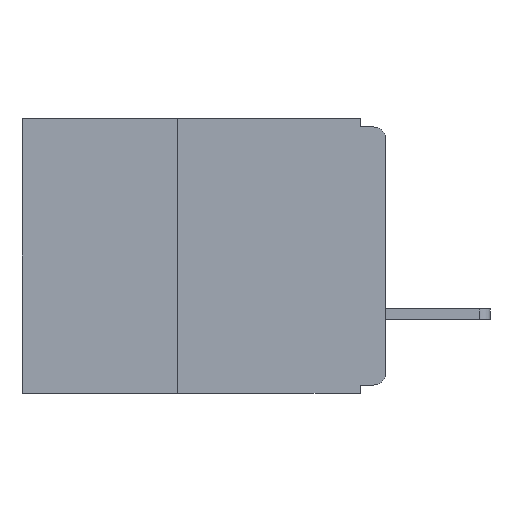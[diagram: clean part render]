
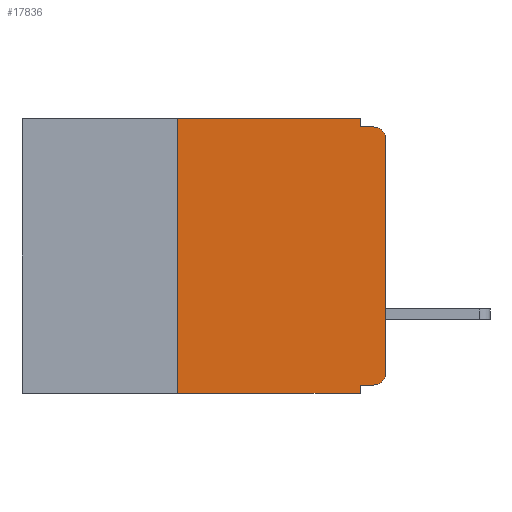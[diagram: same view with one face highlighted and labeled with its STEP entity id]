
A CAD part, left-side view. The second image highlights one B-rep face of the part: STEP entity #17836.
In plain terms, the highlighted planar face has unit normal (-1, 0, 0).
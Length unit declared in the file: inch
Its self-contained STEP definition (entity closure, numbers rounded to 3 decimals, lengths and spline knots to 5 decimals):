
#217 = ORIENTED_EDGE ( 'NONE', *, *, #17724, .F. ) ;
#242 = ORIENTED_EDGE ( 'NONE', *, *, #21918, .T. ) ;
#341 = ORIENTED_EDGE ( 'NONE', *, *, #3918, .T. ) ;
#465 = ORIENTED_EDGE ( 'NONE', *, *, #1792, .T. ) ;
#536 = VECTOR ( 'NONE', #16294, 39.37008 ) ;
#741 = ORIENTED_EDGE ( 'NONE', *, *, #10838, .F. ) ;
#824 = LINE ( 'NONE', #5973, #21567 ) ;
#985 = ORIENTED_EDGE ( 'NONE', *, *, #1573, .F. ) ;
#1011 = VERTEX_POINT ( 'NONE', #6963 ) ;
#1187 = ORIENTED_EDGE ( 'NONE', *, *, #6076, .T. ) ;
#1283 = ORIENTED_EDGE ( 'NONE', *, *, #16368, .F. ) ;
#1501 = DIRECTION ( 'NONE',  ( 0., 0., -1. ) ) ;
#1509 = DIRECTION ( 'NONE',  ( -1., 0., 0. ) ) ;
#1535 = CARTESIAN_POINT ( 'NONE',  ( 0., 0.015, -0.305 ) ) ;
#1573 = EDGE_CURVE ( 'NONE', #5684, #25303, #824, .T. ) ;
#1792 = EDGE_CURVE ( 'NONE', #17069, #1011, #11176, .T. ) ;
#2097 = DIRECTION ( 'NONE',  ( 0., 0., -1. ) ) ;
#2385 = LINE ( 'NONE', #5655, #23067 ) ;
#2975 = VECTOR ( 'NONE', #23339, 39.37008 ) ;
#3246 = VECTOR ( 'NONE', #16067, 39.37008 ) ;
#3507 = CARTESIAN_POINT ( 'NONE',  ( 0., 0., -0.025 ) ) ;
#3577 = CARTESIAN_POINT ( 'NONE',  ( 0., 0., -0.305 ) ) ;
#3665 = EDGE_CURVE ( 'NONE', #7034, #17385, #2385, .T. ) ;
#3918 = EDGE_CURVE ( 'NONE', #24389, #17069, #22154, .T. ) ;
#4003 = PLANE ( 'NONE',  #12230 ) ;
#4044 = CARTESIAN_POINT ( 'NONE',  ( 0., 0.031, -0.33 ) ) ;
#4451 = DIRECTION ( 'NONE',  ( 1., 0., 0. ) ) ;
#4988 = VERTEX_POINT ( 'NONE', #16734 ) ;
#5291 = CARTESIAN_POINT ( 'NONE',  ( 0., 0., -0.01 ) ) ;
#5655 = CARTESIAN_POINT ( 'NONE',  ( 0., 0.031, 0. ) ) ;
#5684 = VERTEX_POINT ( 'NONE', #5942 ) ;
#5814 = DIRECTION ( 'NONE',  ( 0., -1., 0. ) ) ;
#5861 = LINE ( 'NONE', #10238, #536 ) ;
#5942 = CARTESIAN_POINT ( 'NONE',  ( 0., 0.015, -0.32 ) ) ;
#5973 = CARTESIAN_POINT ( 'NONE',  ( 0., 0., -0.32 ) ) ;
#6076 = EDGE_CURVE ( 'NONE', #5684, #24389, #23247, .T. ) ;
#6673 = VECTOR ( 'NONE', #7690, 39.37008 ) ;
#6963 = CARTESIAN_POINT ( 'NONE',  ( 0., 0.015, -0.01 ) ) ;
#7034 = VERTEX_POINT ( 'NONE', #23872 ) ;
#7690 = DIRECTION ( 'NONE',  ( 0., 0., 1. ) ) ;
#8330 = EDGE_LOOP ( 'NONE', ( #341, #465, #1283, #15384, #20646, #217, #242, #741, #985, #1187 ) ) ;
#8595 = LINE ( 'NONE', #4044, #3246 ) ;
#8597 = CARTESIAN_POINT ( 'NONE',  ( 0., 0.031, -0.01 ) ) ;
#8864 = FACE_OUTER_BOUND ( 'NONE', #8330, .T. ) ;
#9011 = EDGE_CURVE ( 'NONE', #11824, #7034, #5861, .T. ) ;
#10238 = CARTESIAN_POINT ( 'NONE',  ( 0., 0.437, 0. ) ) ;
#10838 = EDGE_CURVE ( 'NONE', #25303, #16185, #8595, .T. ) ;
#10985 = DIRECTION ( 'NONE',  ( 0., 1., 0. ) ) ;
#11176 = CIRCLE ( 'NONE', #24838, 0.015 ) ;
#11362 = LINE ( 'NONE', #21753, #6673 ) ;
#11824 = VERTEX_POINT ( 'NONE', #21210 ) ;
#12105 = VECTOR ( 'NONE', #16089, 39.37008 ) ;
#12230 = AXIS2_PLACEMENT_3D ( 'NONE', #16493, #4451, #18567 ) ;
#13435 = AXIS2_PLACEMENT_3D ( 'NONE', #1535, #1509, #1501 ) ;
#15027 = CARTESIAN_POINT ( 'NONE',  ( 0., 0.031, -0.32 ) ) ;
#15384 = ORIENTED_EDGE ( 'NONE', *, *, #3665, .F. ) ;
#16067 = DIRECTION ( 'NONE',  ( 0., 0., -1. ) ) ;
#16089 = DIRECTION ( 'NONE',  ( 0., 0., 1. ) ) ;
#16185 = VERTEX_POINT ( 'NONE', #20790 ) ;
#16294 = DIRECTION ( 'NONE',  ( 0., -1., 0. ) ) ;
#16336 = CARTESIAN_POINT ( 'NONE',  ( 0., 0., 0. ) ) ;
#16368 = EDGE_CURVE ( 'NONE', #17385, #1011, #25436, .T. ) ;
#16493 = CARTESIAN_POINT ( 'NONE',  ( 0., 0.437, 0. ) ) ;
#16734 = CARTESIAN_POINT ( 'NONE',  ( 0., 0.25, -0.33 ) ) ;
#16907 = DIRECTION ( 'NONE',  ( 0., 0., -1. ) ) ;
#17069 = VERTEX_POINT ( 'NONE', #3507 ) ;
#17385 = VERTEX_POINT ( 'NONE', #8597 ) ;
#17724 = EDGE_CURVE ( 'NONE', #4988, #11824, #11362, .T. ) ;
#17836 = ADVANCED_FACE ( 'NONE', ( #8864 ), #4003, .F. ) ;
#18567 = DIRECTION ( 'NONE',  ( 0., 0., -1. ) ) ;
#19270 = VECTOR ( 'NONE', #5814, 39.37008 ) ;
#19917 = CARTESIAN_POINT ( 'NONE',  ( 0., 0.437, -0.33 ) ) ;
#20570 = DIRECTION ( 'NONE',  ( -1., 0., 0. ) ) ;
#20646 = ORIENTED_EDGE ( 'NONE', *, *, #9011, .F. ) ;
#20790 = CARTESIAN_POINT ( 'NONE',  ( 0., 0.031, -0.33 ) ) ;
#21003 = CARTESIAN_POINT ( 'NONE',  ( 0., 0.015, -0.025 ) ) ;
#21210 = CARTESIAN_POINT ( 'NONE',  ( 0., 0.25, 0. ) ) ;
#21567 = VECTOR ( 'NONE', #10985, 39.37008 ) ;
#21753 = CARTESIAN_POINT ( 'NONE',  ( 0., 0.25, -0.33 ) ) ;
#21918 = EDGE_CURVE ( 'NONE', #4988, #16185, #25034, .T. ) ;
#22154 = LINE ( 'NONE', #16336, #12105 ) ;
#23067 = VECTOR ( 'NONE', #2097, 39.37008 ) ;
#23247 = CIRCLE ( 'NONE', #13435, 0.015 ) ;
#23339 = DIRECTION ( 'NONE',  ( 0., -1., 0. ) ) ;
#23872 = CARTESIAN_POINT ( 'NONE',  ( 0., 0.031, 0. ) ) ;
#24389 = VERTEX_POINT ( 'NONE', #3577 ) ;
#24838 = AXIS2_PLACEMENT_3D ( 'NONE', #21003, #20570, #16907 ) ;
#25034 = LINE ( 'NONE', #19917, #19270 ) ;
#25303 = VERTEX_POINT ( 'NONE', #15027 ) ;
#25436 = LINE ( 'NONE', #5291, #2975 ) ;
